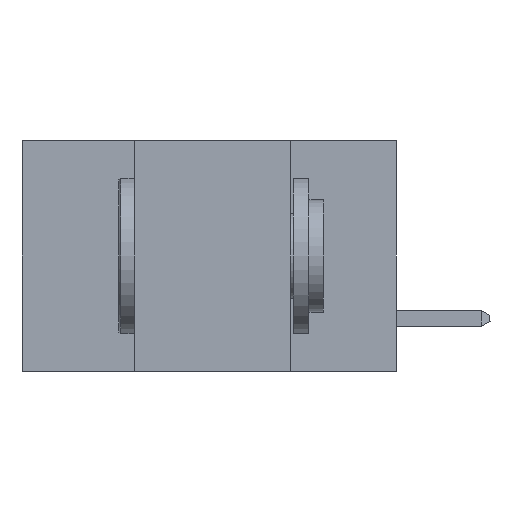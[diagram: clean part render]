
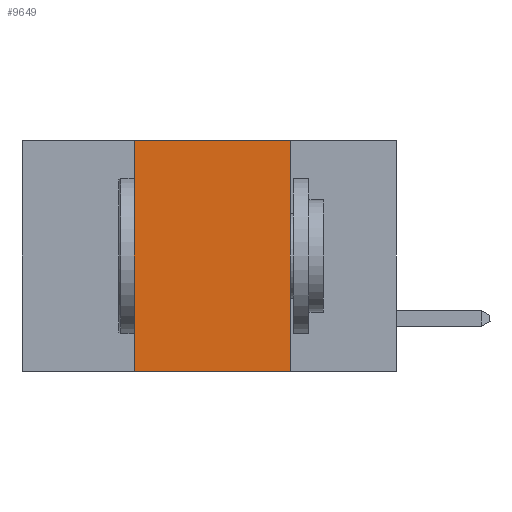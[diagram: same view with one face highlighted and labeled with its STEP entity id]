
A CAD part, left-side view. The second image highlights one B-rep face of the part: STEP entity #9649.
In plain terms, the highlighted planar face has unit normal (-1, 0, 0).
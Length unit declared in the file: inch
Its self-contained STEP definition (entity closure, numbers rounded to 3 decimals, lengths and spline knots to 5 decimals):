
#653 = CARTESIAN_POINT ( 'NONE',  ( 0., 0.42, 0. ) ) ;
#754 = VERTEX_POINT ( 'NONE', #10148 ) ;
#780 = EDGE_LOOP ( 'NONE', ( #16017, #15854, #26011, #26229 ) ) ;
#1186 = DIRECTION ( 'NONE',  ( 0., 0., -1. ) ) ;
#1753 = PLANE ( 'NONE',  #15955 ) ;
#2175 = LINE ( 'NONE', #21836, #8723 ) ;
#2280 = DIRECTION ( 'NONE',  ( 0., 0., -1. ) ) ;
#3634 = VERTEX_POINT ( 'NONE', #8731 ) ;
#3695 = CARTESIAN_POINT ( 'NONE',  ( 0., 0.42, 0. ) ) ;
#3859 = CARTESIAN_POINT ( 'NONE',  ( 0., 0.6, 0. ) ) ;
#4986 = EDGE_CURVE ( 'NONE', #754, #23855, #16718, .T. ) ;
#5118 = EDGE_CURVE ( 'NONE', #23855, #24840, #15069, .T. ) ;
#5247 = CARTESIAN_POINT ( 'NONE',  ( 0., 0.6, -0.37 ) ) ;
#5940 = DIRECTION ( 'NONE',  ( 1., 0., 0. ) ) ;
#8723 = VECTOR ( 'NONE', #1186, 39.37008 ) ;
#8731 = CARTESIAN_POINT ( 'NONE',  ( 0., 0.17, -0.37 ) ) ;
#9505 = VECTOR ( 'NONE', #24098, 39.37008 ) ;
#9649 = ADVANCED_FACE ( 'NONE', ( #14538 ), #1753, .F. ) ;
#10148 = CARTESIAN_POINT ( 'NONE',  ( 0., 0.42, -0.37 ) ) ;
#13789 = VECTOR ( 'NONE', #23824, 39.37008 ) ;
#14538 = FACE_OUTER_BOUND ( 'NONE', #780, .T. ) ;
#15069 = LINE ( 'NONE', #22006, #9505 ) ;
#15854 = ORIENTED_EDGE ( 'NONE', *, *, #5118, .F. ) ;
#15955 = AXIS2_PLACEMENT_3D ( 'NONE', #3859, #5940, #2280 ) ;
#16017 = ORIENTED_EDGE ( 'NONE', *, *, #19243, .F. ) ;
#16254 = LINE ( 'NONE', #5247, #23707 ) ;
#16718 = LINE ( 'NONE', #653, #13789 ) ;
#17455 = CARTESIAN_POINT ( 'NONE',  ( 0., 0.17, 0. ) ) ;
#19243 = EDGE_CURVE ( 'NONE', #24840, #3634, #2175, .T. ) ;
#20969 = EDGE_CURVE ( 'NONE', #754, #3634, #16254, .T. ) ;
#21836 = CARTESIAN_POINT ( 'NONE',  ( 0., 0.17, 0. ) ) ;
#21968 = DIRECTION ( 'NONE',  ( 0., -1., 0. ) ) ;
#22006 = CARTESIAN_POINT ( 'NONE',  ( 0., 0.6, 0. ) ) ;
#23707 = VECTOR ( 'NONE', #21968, 39.37008 ) ;
#23824 = DIRECTION ( 'NONE',  ( 0., 0., 1. ) ) ;
#23855 = VERTEX_POINT ( 'NONE', #3695 ) ;
#24098 = DIRECTION ( 'NONE',  ( 0., -1., 0. ) ) ;
#24840 = VERTEX_POINT ( 'NONE', #17455 ) ;
#26011 = ORIENTED_EDGE ( 'NONE', *, *, #4986, .F. ) ;
#26229 = ORIENTED_EDGE ( 'NONE', *, *, #20969, .T. ) ;
